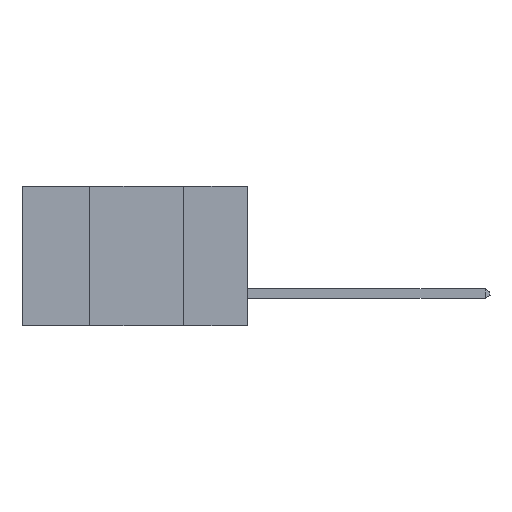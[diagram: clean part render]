
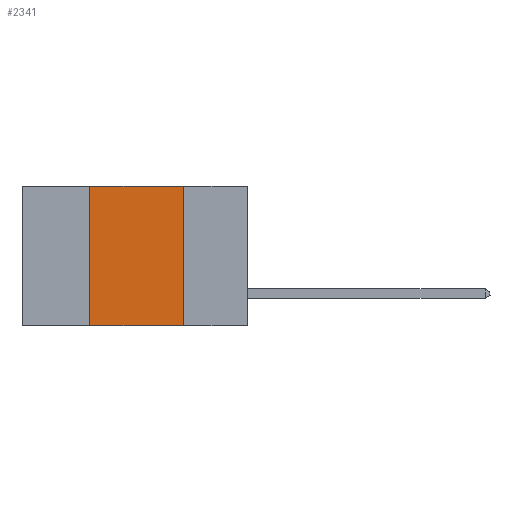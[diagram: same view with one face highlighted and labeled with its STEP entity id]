
A CAD part, left-side view. The second image highlights one B-rep face of the part: STEP entity #2341.
In plain terms, the highlighted planar face has unit normal (-1, 0, 0).
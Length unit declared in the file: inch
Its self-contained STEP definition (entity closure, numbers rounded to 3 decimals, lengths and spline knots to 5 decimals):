
#645 = LINE ( 'NONE', #9278, #12562 ) ;
#1403 = ORIENTED_EDGE ( 'NONE', *, *, #8029, .T. ) ;
#1418 = DIRECTION ( 'NONE',  ( 0., -1., 0. ) ) ;
#1664 = PLANE ( 'NONE',  #23524 ) ;
#2341 = ADVANCED_FACE ( 'NONE', ( #2648 ), #1664, .F. ) ;
#2605 = VECTOR ( 'NONE', #12456, 39.37008 ) ;
#2648 = FACE_OUTER_BOUND ( 'NONE', #7705, .T. ) ;
#3157 = CARTESIAN_POINT ( 'NONE',  ( 0., 0.6, -0.37 ) ) ;
#3415 = CARTESIAN_POINT ( 'NONE',  ( 0., 0.6, 0. ) ) ;
#3738 = ORIENTED_EDGE ( 'NONE', *, *, #23367, .F. ) ;
#4019 = VERTEX_POINT ( 'NONE', #21521 ) ;
#4708 = EDGE_CURVE ( 'NONE', #16606, #22594, #645, .T. ) ;
#5069 = VECTOR ( 'NONE', #20209, 39.37008 ) ;
#7397 = LINE ( 'NONE', #3157, #8599 ) ;
#7705 = EDGE_LOOP ( 'NONE', ( #20607, #13394, #3738, #1403 ) ) ;
#8029 = EDGE_CURVE ( 'NONE', #14306, #4019, #7397, .T. ) ;
#8599 = VECTOR ( 'NONE', #1418, 39.37008 ) ;
#9278 = CARTESIAN_POINT ( 'NONE',  ( 0., 0.6, 0. ) ) ;
#11834 = DIRECTION ( 'NONE',  ( 0., -1., 0. ) ) ;
#12456 = DIRECTION ( 'NONE',  ( 0., 0., 1. ) ) ;
#12562 = VECTOR ( 'NONE', #11834, 39.37008 ) ;
#12964 = CARTESIAN_POINT ( 'NONE',  ( 0., 0.42, 0. ) ) ;
#13394 = ORIENTED_EDGE ( 'NONE', *, *, #4708, .F. ) ;
#13602 = CARTESIAN_POINT ( 'NONE',  ( 0., 0.17, 0. ) ) ;
#14225 = CARTESIAN_POINT ( 'NONE',  ( 0., 0.42, 0. ) ) ;
#14306 = VERTEX_POINT ( 'NONE', #22980 ) ;
#15387 = DIRECTION ( 'NONE',  ( 0., 0., -1. ) ) ;
#15565 = DIRECTION ( 'NONE',  ( 1., 0., 0. ) ) ;
#16606 = VERTEX_POINT ( 'NONE', #12964 ) ;
#18225 = CARTESIAN_POINT ( 'NONE',  ( 0., 0.17, 0. ) ) ;
#20209 = DIRECTION ( 'NONE',  ( 0., 0., -1. ) ) ;
#20464 = LINE ( 'NONE', #14225, #2605 ) ;
#20607 = ORIENTED_EDGE ( 'NONE', *, *, #20901, .F. ) ;
#20852 = LINE ( 'NONE', #18225, #5069 ) ;
#20901 = EDGE_CURVE ( 'NONE', #22594, #4019, #20852, .T. ) ;
#21521 = CARTESIAN_POINT ( 'NONE',  ( 0., 0.17, -0.37 ) ) ;
#22594 = VERTEX_POINT ( 'NONE', #13602 ) ;
#22980 = CARTESIAN_POINT ( 'NONE',  ( 0., 0.42, -0.37 ) ) ;
#23367 = EDGE_CURVE ( 'NONE', #14306, #16606, #20464, .T. ) ;
#23524 = AXIS2_PLACEMENT_3D ( 'NONE', #3415, #15565, #15387 ) ;
